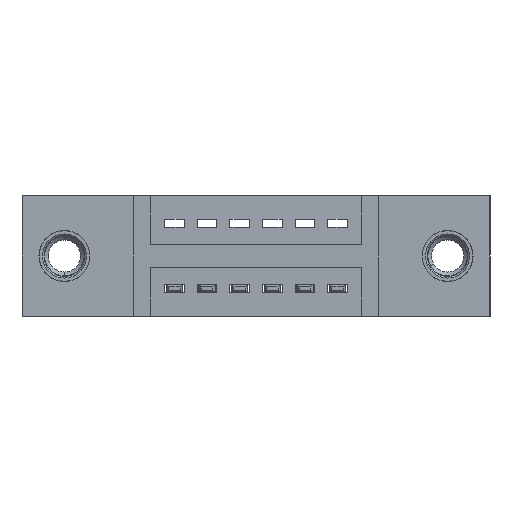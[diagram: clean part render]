
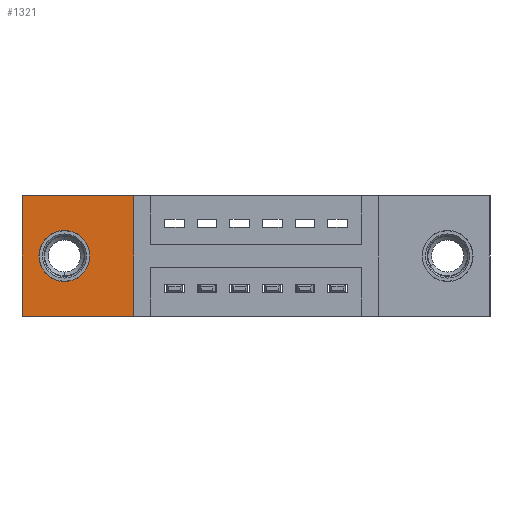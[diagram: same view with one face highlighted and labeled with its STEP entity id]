
A CAD part, front view. The second image highlights one B-rep face of the part: STEP entity #1321.
In plain terms, the highlighted planar face has unit normal (0, -1, 0).
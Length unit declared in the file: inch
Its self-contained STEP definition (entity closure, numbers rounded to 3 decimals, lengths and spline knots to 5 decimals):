
#108 = CARTESIAN_POINT ( 'NONE',  ( 0., 0.17, -0.37 ) ) ;
#540 = VERTEX_POINT ( 'NONE', #10047 ) ;
#638 = DIRECTION ( 'NONE',  ( 0., 0., -1. ) ) ;
#784 = VECTOR ( 'NONE', #4288, 39.37008 ) ;
#842 = EDGE_CURVE ( 'NONE', #7204, #10295, #8377, .T. ) ;
#1064 = CARTESIAN_POINT ( 'NONE',  ( 0.13, 0.17, -0.263 ) ) ;
#1198 = EDGE_LOOP ( 'NONE', ( #7656, #3793 ) ) ;
#1321 = ADVANCED_FACE ( 'NONE', ( #10049, #1528 ), #9224, .T. ) ;
#1528 = FACE_OUTER_BOUND ( 'NONE', #4385, .T. ) ;
#1935 = DIRECTION ( 'NONE',  ( 0., -1., 0. ) ) ;
#2049 = VECTOR ( 'NONE', #638, 39.37008 ) ;
#2271 = VERTEX_POINT ( 'NONE', #8025 ) ;
#2451 = CARTESIAN_POINT ( 'NONE',  ( 0., 0.17, 0. ) ) ;
#2863 = DIRECTION ( 'NONE',  ( 1., 0., 0. ) ) ;
#2986 = EDGE_CURVE ( 'NONE', #9528, #540, #3618, .T. ) ;
#3103 = ORIENTED_EDGE ( 'NONE', *, *, #2986, .T. ) ;
#3422 = AXIS2_PLACEMENT_3D ( 'NONE', #6984, #1935, #7729 ) ;
#3613 = LINE ( 'NONE', #108, #7410 ) ;
#3618 = LINE ( 'NONE', #5009, #9361 ) ;
#3793 = ORIENTED_EDGE ( 'NONE', *, *, #842, .F. ) ;
#4288 = DIRECTION ( 'NONE',  ( 0., 0., 1. ) ) ;
#4320 = EDGE_CURVE ( 'NONE', #540, #2271, #6550, .T. ) ;
#4385 = EDGE_LOOP ( 'NONE', ( #10159, #8961, #7229, #3103 ) ) ;
#4608 = EDGE_CURVE ( 'NONE', #10295, #7204, #8380, .T. ) ;
#4640 = AXIS2_PLACEMENT_3D ( 'NONE', #9925, #9213, #9210 ) ;
#4784 = DIRECTION ( 'NONE',  ( 0., 0., -1. ) ) ;
#4807 = DIRECTION ( 'NONE',  ( 0., -1., 0. ) ) ;
#4811 = CARTESIAN_POINT ( 'NONE',  ( 0.13, 0.17, -0.185 ) ) ;
#5009 = CARTESIAN_POINT ( 'NONE',  ( 0., 0.17, 0. ) ) ;
#5851 = EDGE_CURVE ( 'NONE', #10068, #9528, #9480, .T. ) ;
#5906 = DIRECTION ( 'NONE',  ( -1., 0., 0. ) ) ;
#6503 = EDGE_CURVE ( 'NONE', #2271, #10068, #3613, .T. ) ;
#6514 = CARTESIAN_POINT ( 'NONE',  ( 0.13, 0.17, -0.107 ) ) ;
#6550 = LINE ( 'NONE', #2451, #2049 ) ;
#6984 = CARTESIAN_POINT ( 'NONE',  ( 0.13, 0.17, -0.185 ) ) ;
#7093 = CARTESIAN_POINT ( 'NONE',  ( 0.3425, 0.17, 0. ) ) ;
#7204 = VERTEX_POINT ( 'NONE', #1064 ) ;
#7229 = ORIENTED_EDGE ( 'NONE', *, *, #5851, .T. ) ;
#7410 = VECTOR ( 'NONE', #2863, 39.37008 ) ;
#7656 = ORIENTED_EDGE ( 'NONE', *, *, #4608, .F. ) ;
#7729 = DIRECTION ( 'NONE',  ( 0., 0., -1. ) ) ;
#8025 = CARTESIAN_POINT ( 'NONE',  ( 0., 0.17, -0.37 ) ) ;
#8377 = CIRCLE ( 'NONE', #9306, 0.078 ) ;
#8380 = CIRCLE ( 'NONE', #3422, 0.078 ) ;
#8954 = CARTESIAN_POINT ( 'NONE',  ( 0.3425, 0.17, 0. ) ) ;
#8961 = ORIENTED_EDGE ( 'NONE', *, *, #6503, .T. ) ;
#9210 = DIRECTION ( 'NONE',  ( 0., 0., -1. ) ) ;
#9213 = DIRECTION ( 'NONE',  ( 0., -1., 0. ) ) ;
#9224 = PLANE ( 'NONE',  #4640 ) ;
#9306 = AXIS2_PLACEMENT_3D ( 'NONE', #4811, #4807, #4784 ) ;
#9361 = VECTOR ( 'NONE', #5906, 39.37008 ) ;
#9480 = LINE ( 'NONE', #8954, #784 ) ;
#9528 = VERTEX_POINT ( 'NONE', #7093 ) ;
#9925 = CARTESIAN_POINT ( 'NONE',  ( 0., 0.17, -0.37 ) ) ;
#9930 = CARTESIAN_POINT ( 'NONE',  ( 0.3425, 0.17, -0.37 ) ) ;
#10047 = CARTESIAN_POINT ( 'NONE',  ( 0., 0.17, 0. ) ) ;
#10049 = FACE_BOUND ( 'NONE', #1198, .T. ) ;
#10068 = VERTEX_POINT ( 'NONE', #9930 ) ;
#10159 = ORIENTED_EDGE ( 'NONE', *, *, #4320, .T. ) ;
#10295 = VERTEX_POINT ( 'NONE', #6514 ) ;
